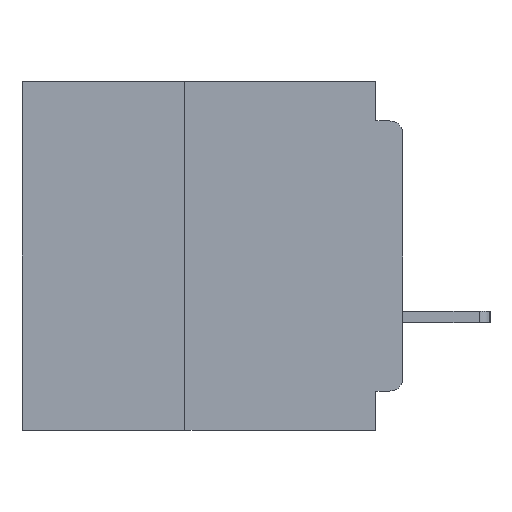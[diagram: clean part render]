
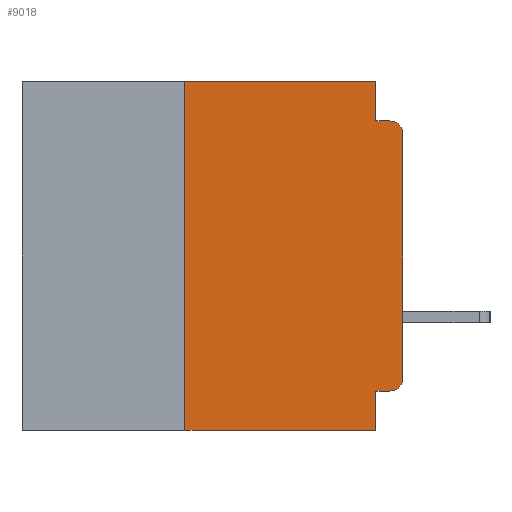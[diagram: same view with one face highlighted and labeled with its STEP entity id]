
A CAD part, left-side view. The second image highlights one B-rep face of the part: STEP entity #9018.
In plain terms, the highlighted planar face has unit normal (-1, 0, 0).
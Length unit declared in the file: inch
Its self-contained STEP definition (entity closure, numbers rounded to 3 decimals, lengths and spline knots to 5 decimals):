
#349 = ORIENTED_EDGE ( 'NONE', *, *, #936, .F. ) ;
#380 = CARTESIAN_POINT ( 'NONE',  ( 0., 0.015, -0.06 ) ) ;
#504 = EDGE_CURVE ( 'NONE', #31671, #28287, #17668, .T. ) ;
#770 = AXIS2_PLACEMENT_3D ( 'NONE', #380, #1035, #786 ) ;
#786 = DIRECTION ( 'NONE',  ( 0., 0., -1. ) ) ;
#936 = EDGE_CURVE ( 'NONE', #18081, #35721, #2670, .T. ) ;
#1035 = DIRECTION ( 'NONE',  ( -1., 0., 0. ) ) ;
#1755 = DIRECTION ( 'NONE',  ( 0., 1., 0. ) ) ;
#2472 = ORIENTED_EDGE ( 'NONE', *, *, #29086, .T. ) ;
#2670 = LINE ( 'NONE', #25215, #33315 ) ;
#4968 = AXIS2_PLACEMENT_3D ( 'NONE', #9374, #30052, #12358 ) ;
#6701 = VECTOR ( 'NONE', #19368, 39.37008 ) ;
#6883 = CARTESIAN_POINT ( 'NONE',  ( 0., 0., -0.045 ) ) ;
#6984 = ORIENTED_EDGE ( 'NONE', *, *, #33783, .T. ) ;
#7023 = LINE ( 'NONE', #21870, #29710 ) ;
#7130 = EDGE_CURVE ( 'NONE', #9961, #35560, #15553, .T. ) ;
#7412 = VERTEX_POINT ( 'NONE', #19333 ) ;
#7540 = VECTOR ( 'NONE', #18576, 39.37008 ) ;
#7701 = CARTESIAN_POINT ( 'NONE',  ( 0., 0., 0. ) ) ;
#7825 = LINE ( 'NONE', #27844, #38271 ) ;
#7959 = VECTOR ( 'NONE', #9917, 39.37008 ) ;
#8304 = CIRCLE ( 'NONE', #4968, 0.015 ) ;
#8485 = ORIENTED_EDGE ( 'NONE', *, *, #10703, .T. ) ;
#8531 = EDGE_CURVE ( 'NONE', #35560, #28287, #24664, .T. ) ;
#8719 = AXIS2_PLACEMENT_3D ( 'NONE', #32732, #15074, #35690 ) ;
#9018 = ADVANCED_FACE ( 'NONE', ( #20534 ), #12081, .F. ) ;
#9096 = DIRECTION ( 'NONE',  ( 0., 0., -1. ) ) ;
#9374 = CARTESIAN_POINT ( 'NONE',  ( 0., 0.015, -0.34 ) ) ;
#9660 = CARTESIAN_POINT ( 'NONE',  ( 0., 0.25, -0.4 ) ) ;
#9917 = DIRECTION ( 'NONE',  ( 0., -1., 0. ) ) ;
#9939 = DIRECTION ( 'NONE',  ( 0., -1., 0. ) ) ;
#9961 = VERTEX_POINT ( 'NONE', #32408 ) ;
#10703 = EDGE_CURVE ( 'NONE', #18081, #14180, #8304, .T. ) ;
#10848 = EDGE_CURVE ( 'NONE', #19058, #9961, #7825, .T. ) ;
#11716 = ORIENTED_EDGE ( 'NONE', *, *, #10848, .F. ) ;
#12081 = PLANE ( 'NONE',  #8719 ) ;
#12358 = DIRECTION ( 'NONE',  ( 0., 0., -1. ) ) ;
#12551 = EDGE_CURVE ( 'NONE', #35721, #7412, #38119, .T. ) ;
#12874 = ORIENTED_EDGE ( 'NONE', *, *, #12551, .F. ) ;
#14147 = VERTEX_POINT ( 'NONE', #9660 ) ;
#14180 = VERTEX_POINT ( 'NONE', #18725 ) ;
#14891 = ORIENTED_EDGE ( 'NONE', *, *, #7130, .F. ) ;
#15074 = DIRECTION ( 'NONE',  ( 1., 0., 0. ) ) ;
#15458 = LINE ( 'NONE', #15620, #7540 ) ;
#15553 = LINE ( 'NONE', #35698, #30320 ) ;
#15620 = CARTESIAN_POINT ( 'NONE',  ( 0., 0.25, -0.4 ) ) ;
#16089 = CARTESIAN_POINT ( 'NONE',  ( 0., 0.015, -0.355 ) ) ;
#16328 = ORIENTED_EDGE ( 'NONE', *, *, #504, .T. ) ;
#16414 = CARTESIAN_POINT ( 'NONE',  ( 0., 0.031, -0.4 ) ) ;
#17668 = CIRCLE ( 'NONE', #770, 0.015 ) ;
#18081 = VERTEX_POINT ( 'NONE', #16089 ) ;
#18576 = DIRECTION ( 'NONE',  ( 0., 0., 1. ) ) ;
#18725 = CARTESIAN_POINT ( 'NONE',  ( 0., 0., -0.34 ) ) ;
#18877 = CARTESIAN_POINT ( 'NONE',  ( 0., 0.031, -0.045 ) ) ;
#19058 = VERTEX_POINT ( 'NONE', #35723 ) ;
#19156 = EDGE_CURVE ( 'NONE', #14147, #19058, #15458, .T. ) ;
#19169 = ORIENTED_EDGE ( 'NONE', *, *, #19156, .F. ) ;
#19333 = CARTESIAN_POINT ( 'NONE',  ( 0., 0.031, -0.4 ) ) ;
#19368 = DIRECTION ( 'NONE',  ( 0., 0., -1. ) ) ;
#19648 = DIRECTION ( 'NONE',  ( 0., 0., 1. ) ) ;
#20534 = FACE_OUTER_BOUND ( 'NONE', #34946, .T. ) ;
#21870 = CARTESIAN_POINT ( 'NONE',  ( 0., 0.437, -0.4 ) ) ;
#22195 = CARTESIAN_POINT ( 'NONE',  ( 0., 0., -0.06 ) ) ;
#24664 = LINE ( 'NONE', #6883, #7959 ) ;
#25041 = DIRECTION ( 'NONE',  ( 0., -1., 0. ) ) ;
#25215 = CARTESIAN_POINT ( 'NONE',  ( 0., 0., -0.355 ) ) ;
#27844 = CARTESIAN_POINT ( 'NONE',  ( 0., 0.437, 0. ) ) ;
#28287 = VERTEX_POINT ( 'NONE', #37355 ) ;
#28400 = CARTESIAN_POINT ( 'NONE',  ( 0., 0.031, -0.355 ) ) ;
#29086 = EDGE_CURVE ( 'NONE', #14147, #7412, #7023, .T. ) ;
#29710 = VECTOR ( 'NONE', #9939, 39.37008 ) ;
#30052 = DIRECTION ( 'NONE',  ( -1., 0., 0. ) ) ;
#30320 = VECTOR ( 'NONE', #9096, 39.37008 ) ;
#30599 = ORIENTED_EDGE ( 'NONE', *, *, #8531, .F. ) ;
#31671 = VERTEX_POINT ( 'NONE', #22195 ) ;
#32408 = CARTESIAN_POINT ( 'NONE',  ( 0., 0.031, 0. ) ) ;
#32732 = CARTESIAN_POINT ( 'NONE',  ( 0., 0.437, 0. ) ) ;
#33315 = VECTOR ( 'NONE', #1755, 39.37008 ) ;
#33783 = EDGE_CURVE ( 'NONE', #14180, #31671, #35279, .T. ) ;
#34378 = VECTOR ( 'NONE', #19648, 39.37008 ) ;
#34946 = EDGE_LOOP ( 'NONE', ( #6984, #16328, #30599, #14891, #11716, #19169, #2472, #12874, #349, #8485 ) ) ;
#35279 = LINE ( 'NONE', #7701, #34378 ) ;
#35560 = VERTEX_POINT ( 'NONE', #18877 ) ;
#35690 = DIRECTION ( 'NONE',  ( 0., 0., -1. ) ) ;
#35698 = CARTESIAN_POINT ( 'NONE',  ( 0., 0.031, 0. ) ) ;
#35721 = VERTEX_POINT ( 'NONE', #28400 ) ;
#35723 = CARTESIAN_POINT ( 'NONE',  ( 0., 0.25, 0. ) ) ;
#37355 = CARTESIAN_POINT ( 'NONE',  ( 0., 0.015, -0.045 ) ) ;
#38119 = LINE ( 'NONE', #16414, #6701 ) ;
#38271 = VECTOR ( 'NONE', #25041, 39.37008 ) ;
